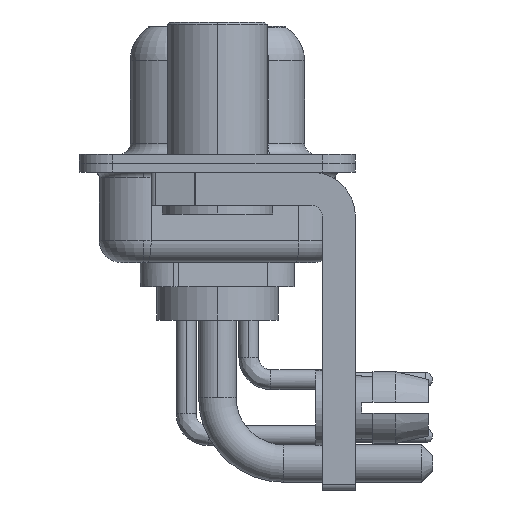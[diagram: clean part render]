
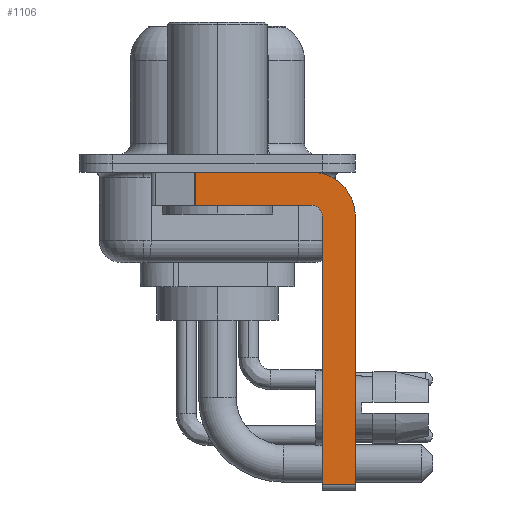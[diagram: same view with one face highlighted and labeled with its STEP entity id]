
A CAD part, left-side view. The second image highlights one B-rep face of the part: STEP entity #1106.
In plain terms, the highlighted planar face has unit normal (-1, 0, 0).
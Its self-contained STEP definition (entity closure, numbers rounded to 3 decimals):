
#279 = VECTOR ( 'NONE', #4972, 1000. ) ;
#334 = EDGE_CURVE ( 'NONE', #7380, #8483, #6147, .T. ) ;
#338 = CIRCLE ( 'NONE', #7624, 2. ) ;
#1106 = ADVANCED_FACE ( 'NONE', ( #12567 ), #3677, .F. ) ;
#1467 = CARTESIAN_POINT ( 'NONE',  ( -2.9, -4.25, -2.4 ) ) ;
#1797 = ORIENTED_EDGE ( 'NONE', *, *, #334, .F. ) ;
#1842 = DIRECTION ( 'NONE',  ( 0., 0., -1. ) ) ;
#2012 = VERTEX_POINT ( 'NONE', #17262 ) ;
#2291 = DIRECTION ( 'NONE',  ( 0., 0., 1. ) ) ;
#2587 = CARTESIAN_POINT ( 'NONE',  ( -2.9, -4.25, -1.9 ) ) ;
#2952 = LINE ( 'NONE', #4684, #13669 ) ;
#3677 = PLANE ( 'NONE',  #6804 ) ;
#3779 = CARTESIAN_POINT ( 'NONE',  ( -2.9, -4.25, -2.4 ) ) ;
#4684 = CARTESIAN_POINT ( 'NONE',  ( -2.9, 3., -0.4 ) ) ;
#4972 = DIRECTION ( 'NONE',  ( 0., -1., 0. ) ) ;
#5130 = DIRECTION ( 'NONE',  ( 0., 0., -1. ) ) ;
#5163 = ORIENTED_EDGE ( 'NONE', *, *, #11989, .F. ) ;
#5325 = VECTOR ( 'NONE', #16347, 1000. ) ;
#5712 = CARTESIAN_POINT ( 'NONE',  ( -2.9, -6.25, -2.4 ) ) ;
#6007 = LINE ( 'NONE', #2587, #20334 ) ;
#6031 = CARTESIAN_POINT ( 'NONE',  ( -2.9, -6.25, -2.4 ) ) ;
#6147 = LINE ( 'NONE', #6031, #5325 ) ;
#6165 = EDGE_CURVE ( 'NONE', #12477, #17598, #2952, .T. ) ;
#6275 = ORIENTED_EDGE ( 'NONE', *, *, #20236, .F. ) ;
#6676 = LINE ( 'NONE', #20609, #279 ) ;
#6804 = AXIS2_PLACEMENT_3D ( 'NONE', #15931, #7086, #1842 ) ;
#7086 = DIRECTION ( 'NONE',  ( 1., 0., 0. ) ) ;
#7380 = VERTEX_POINT ( 'NONE', #5712 ) ;
#7624 = AXIS2_PLACEMENT_3D ( 'NONE', #1467, #20770, #5130 ) ;
#7793 = ORIENTED_EDGE ( 'NONE', *, *, #11602, .F. ) ;
#7885 = DIRECTION ( 'NONE',  ( 0., 0., 1. ) ) ;
#8152 = CARTESIAN_POINT ( 'NONE',  ( -2.9, 0.978, -1.9 ) ) ;
#8264 = LINE ( 'NONE', #8152, #16831 ) ;
#8483 = VERTEX_POINT ( 'NONE', #13606 ) ;
#8842 = ORIENTED_EDGE ( 'NONE', *, *, #19143, .T. ) ;
#9869 = CARTESIAN_POINT ( 'NONE',  ( -2.9, -4.25, -1.9 ) ) ;
#10161 = AXIS2_PLACEMENT_3D ( 'NONE', #3779, #17717, #2291 ) ;
#10190 = ORIENTED_EDGE ( 'NONE', *, *, #12797, .T. ) ;
#10897 = ORIENTED_EDGE ( 'NONE', *, *, #6165, .F. ) ;
#10999 = VERTEX_POINT ( 'NONE', #19036 ) ;
#11602 = EDGE_CURVE ( 'NONE', #2012, #20343, #17136, .T. ) ;
#11989 = EDGE_CURVE ( 'NONE', #17598, #7380, #338, .T. ) ;
#12477 = VERTEX_POINT ( 'NONE', #16202 ) ;
#12567 = FACE_OUTER_BOUND ( 'NONE', #14767, .T. ) ;
#12797 = EDGE_CURVE ( 'NONE', #12477, #16672, #8264, .T. ) ;
#13435 = CARTESIAN_POINT ( 'NONE',  ( -2.9, -4.25, -0.4 ) ) ;
#13606 = CARTESIAN_POINT ( 'NONE',  ( -2.9, -6.25, -14.55 ) ) ;
#13669 = VECTOR ( 'NONE', #14976, 1000. ) ;
#13855 = CARTESIAN_POINT ( 'NONE',  ( -2.9, 0.978, -1.9 ) ) ;
#14767 = EDGE_LOOP ( 'NONE', ( #10897, #10190, #6275, #7793, #19079, #8842, #1797, #5163 ) ) ;
#14976 = DIRECTION ( 'NONE',  ( 0., -1., 0. ) ) ;
#15931 = CARTESIAN_POINT ( 'NONE',  ( -2.9, -4.25, -2.4 ) ) ;
#16202 = CARTESIAN_POINT ( 'NONE',  ( -2.9, 0.978, -0.4 ) ) ;
#16347 = DIRECTION ( 'NONE',  ( 0., 0., -1. ) ) ;
#16434 = DIRECTION ( 'NONE',  ( 0., 1., 0. ) ) ;
#16672 = VERTEX_POINT ( 'NONE', #13855 ) ;
#16831 = VECTOR ( 'NONE', #20390, 1000. ) ;
#17136 = CIRCLE ( 'NONE', #10161, 0.5 ) ;
#17262 = CARTESIAN_POINT ( 'NONE',  ( -2.9, -4.75, -2.4 ) ) ;
#17598 = VERTEX_POINT ( 'NONE', #13435 ) ;
#17717 = DIRECTION ( 'NONE',  ( -1., 0., 0. ) ) ;
#18183 = VECTOR ( 'NONE', #7885, 1000. ) ;
#19036 = CARTESIAN_POINT ( 'NONE',  ( -2.9, -4.75, -14.55 ) ) ;
#19079 = ORIENTED_EDGE ( 'NONE', *, *, #21246, .F. ) ;
#19143 = EDGE_CURVE ( 'NONE', #10999, #8483, #6676, .T. ) ;
#20015 = CARTESIAN_POINT ( 'NONE',  ( -2.9, -4.75, -14.8 ) ) ;
#20236 = EDGE_CURVE ( 'NONE', #20343, #16672, #6007, .T. ) ;
#20334 = VECTOR ( 'NONE', #16434, 1000. ) ;
#20343 = VERTEX_POINT ( 'NONE', #9869 ) ;
#20390 = DIRECTION ( 'NONE',  ( 0., 0., -1. ) ) ;
#20609 = CARTESIAN_POINT ( 'NONE',  ( -2.9, -4.25, -14.55 ) ) ;
#20770 = DIRECTION ( 'NONE',  ( 1., 0., 0. ) ) ;
#21246 = EDGE_CURVE ( 'NONE', #10999, #2012, #21389, .T. ) ;
#21389 = LINE ( 'NONE', #20015, #18183 ) ;
